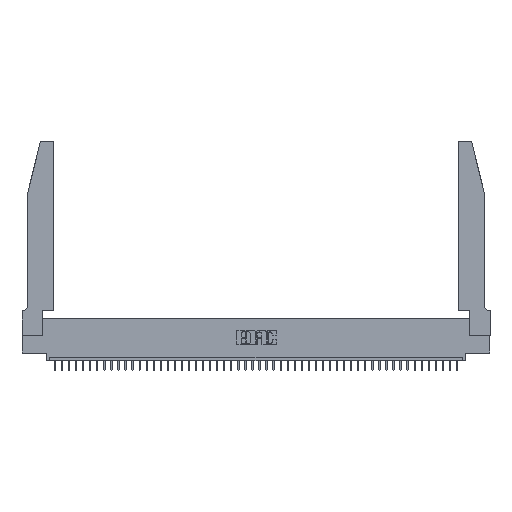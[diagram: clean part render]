
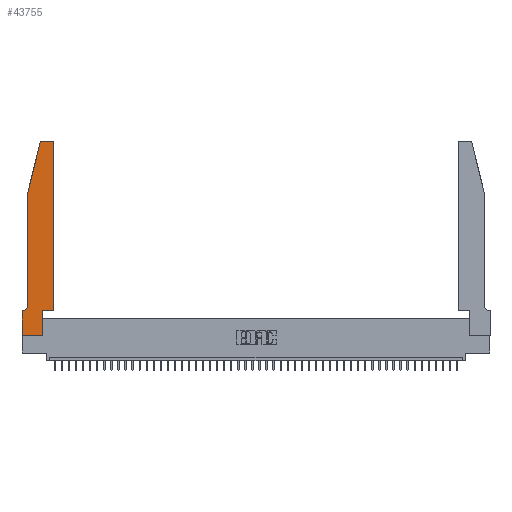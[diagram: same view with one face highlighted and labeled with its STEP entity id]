
A CAD part, top view. The second image highlights one B-rep face of the part: STEP entity #43755.
In plain terms, the highlighted planar face has unit normal (0, 0, 1).
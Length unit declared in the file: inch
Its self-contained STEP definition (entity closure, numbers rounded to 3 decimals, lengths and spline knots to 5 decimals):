
#264 = CARTESIAN_POINT ( 'NONE',  ( 0.4505, 0.35, 0.37 ) ) ;
#1302 = EDGE_CURVE ( 'NONE', #27855, #21250, #41207, .T. ) ;
#1537 = CARTESIAN_POINT ( 'NONE',  ( 0.2865, 0.35, 0.37 ) ) ;
#1675 = ORIENTED_EDGE ( 'NONE', *, *, #24866, .T. ) ;
#2288 = LINE ( 'NONE', #20576, #5714 ) ;
#2392 = ORIENTED_EDGE ( 'NONE', *, *, #37193, .T. ) ;
#2467 = DIRECTION ( 'NONE',  ( 1., 0., 0. ) ) ;
#2756 = DIRECTION ( 'NONE',  ( 0., 1., 0. ) ) ;
#2784 = CARTESIAN_POINT ( 'NONE',  ( 0., 0.35, 0.37 ) ) ;
#2833 = DIRECTION ( 'NONE',  ( 0., 1., 0. ) ) ;
#2867 = VERTEX_POINT ( 'NONE', #39076 ) ;
#2990 = LINE ( 'NONE', #38467, #31828 ) ;
#3200 = EDGE_CURVE ( 'NONE', #21250, #3592, #3771, .T. ) ;
#3344 = LINE ( 'NONE', #264, #46475 ) ;
#3357 = ORIENTED_EDGE ( 'NONE', *, *, #3200, .T. ) ;
#3592 = VERTEX_POINT ( 'NONE', #2784 ) ;
#3771 = LINE ( 'NONE', #38771, #34557 ) ;
#5037 = CARTESIAN_POINT ( 'NONE',  ( 0.0755, 2., 0.37 ) ) ;
#5418 = EDGE_CURVE ( 'NONE', #41456, #9614, #2288, .T. ) ;
#5714 = VECTOR ( 'NONE', #16613, 39.37008 ) ;
#5960 = LINE ( 'NONE', #45240, #11482 ) ;
#6958 = CARTESIAN_POINT ( 'NONE',  ( 0.284, 2.75, 0.37 ) ) ;
#9614 = VERTEX_POINT ( 'NONE', #36495 ) ;
#10933 = AXIS2_PLACEMENT_3D ( 'NONE', #23113, #23816, #38168 ) ;
#11343 = CIRCLE ( 'NONE', #37610, 0.03 ) ;
#11482 = VECTOR ( 'NONE', #2467, 39.37008 ) ;
#12267 = EDGE_LOOP ( 'NONE', ( #12749, #43530, #13342, #14851, #34036, #3357, #14149, #40280, #2392, #42584, #1675, #34532 ) ) ;
#12749 = ORIENTED_EDGE ( 'NONE', *, *, #28245, .T. ) ;
#12794 = EDGE_CURVE ( 'NONE', #17202, #34576, #3344, .T. ) ;
#12832 = AXIS2_PLACEMENT_3D ( 'NONE', #39432, #14291, #42969 ) ;
#13342 = ORIENTED_EDGE ( 'NONE', *, *, #5418, .T. ) ;
#13403 = VECTOR ( 'NONE', #40559, 39.37008 ) ;
#14149 = ORIENTED_EDGE ( 'NONE', *, *, #24190, .T. ) ;
#14291 = DIRECTION ( 'NONE',  ( 0., 0., 1. ) ) ;
#14851 = ORIENTED_EDGE ( 'NONE', *, *, #39822, .T. ) ;
#15056 = LINE ( 'NONE', #36428, #31975 ) ;
#16613 = DIRECTION ( 'NONE',  ( -0.239, -0.971, 0. ) ) ;
#17202 = VERTEX_POINT ( 'NONE', #1537 ) ;
#17816 = FACE_OUTER_BOUND ( 'NONE', #12267, .T. ) ;
#18684 = EDGE_CURVE ( 'NONE', #46118, #2867, #5960, .T. ) ;
#18891 = CARTESIAN_POINT ( 'NONE',  ( 0.0755, 0.42, 0.37 ) ) ;
#20576 = CARTESIAN_POINT ( 'NONE',  ( 0.0755, 2., 0.37 ) ) ;
#20604 = CARTESIAN_POINT ( 'NONE',  ( 0.4505, 0.35, 0.37 ) ) ;
#21250 = VERTEX_POINT ( 'NONE', #24347 ) ;
#21313 = VERTEX_POINT ( 'NONE', #6958 ) ;
#21409 = CARTESIAN_POINT ( 'NONE',  ( 0.2605, 2.75, 0.37 ) ) ;
#22088 = LINE ( 'NONE', #21409, #25911 ) ;
#22305 = DIRECTION ( 'NONE',  ( 0., -1., 0. ) ) ;
#23113 = CARTESIAN_POINT ( 'NONE',  ( 0.4205, 2.72, 0.37 ) ) ;
#23816 = DIRECTION ( 'NONE',  ( 0., 0., 1. ) ) ;
#24071 = EDGE_CURVE ( 'NONE', #45318, #38847, #34950, .T. ) ;
#24190 = EDGE_CURVE ( 'NONE', #3592, #46118, #15056, .T. ) ;
#24347 = CARTESIAN_POINT ( 'NONE',  ( 0.0055, 0.35, 0.37 ) ) ;
#24866 = EDGE_CURVE ( 'NONE', #34576, #45318, #2990, .T. ) ;
#25402 = DIRECTION ( 'NONE',  ( 1., 0., 0. ) ) ;
#25911 = VECTOR ( 'NONE', #35755, 39.37008 ) ;
#26119 = CARTESIAN_POINT ( 'NONE',  ( 0.4505, 2.72, 0.37 ) ) ;
#27855 = VERTEX_POINT ( 'NONE', #18891 ) ;
#28013 = CARTESIAN_POINT ( 'NONE',  ( 0.25487, 2.72718, 0.37 ) ) ;
#28245 = EDGE_CURVE ( 'NONE', #38847, #21313, #22088, .T. ) ;
#28891 = DIRECTION ( 'NONE',  ( -1., 0., 0. ) ) ;
#29204 = CARTESIAN_POINT ( 'NONE',  ( 0.4205, 2.75, 0.37 ) ) ;
#29949 = DIRECTION ( 'NONE',  ( -1., 0., 0. ) ) ;
#30561 = DIRECTION ( 'NONE',  ( 0., 0., 1. ) ) ;
#31332 = CARTESIAN_POINT ( 'NONE',  ( 0., 0., 0.37 ) ) ;
#31828 = VECTOR ( 'NONE', #2756, 39.37008 ) ;
#31975 = VECTOR ( 'NONE', #22305, 39.37008 ) ;
#34036 = ORIENTED_EDGE ( 'NONE', *, *, #1302, .T. ) ;
#34532 = ORIENTED_EDGE ( 'NONE', *, *, #24071, .T. ) ;
#34557 = VECTOR ( 'NONE', #28891, 39.37008 ) ;
#34576 = VERTEX_POINT ( 'NONE', #20604 ) ;
#34950 = CIRCLE ( 'NONE', #10933, 0.03 ) ;
#35016 = LINE ( 'NONE', #46083, #40634 ) ;
#35755 = DIRECTION ( 'NONE',  ( -1., 0., 0. ) ) ;
#36428 = CARTESIAN_POINT ( 'NONE',  ( 0., 0., 0.37 ) ) ;
#36495 = CARTESIAN_POINT ( 'NONE',  ( 0.0755, 2., 0.37 ) ) ;
#36989 = CARTESIAN_POINT ( 'NONE',  ( 0.0055, 0.42, 0.37 ) ) ;
#37030 = EDGE_CURVE ( 'NONE', #21313, #41456, #11343, .T. ) ;
#37193 = EDGE_CURVE ( 'NONE', #2867, #17202, #35016, .T. ) ;
#37380 = CARTESIAN_POINT ( 'NONE',  ( 0.284, 2.72, 0.37 ) ) ;
#37610 = AXIS2_PLACEMENT_3D ( 'NONE', #37380, #30561, #44678 ) ;
#38168 = DIRECTION ( 'NONE',  ( 1., 0., 0. ) ) ;
#38467 = CARTESIAN_POINT ( 'NONE',  ( 0.4505, 0.35, 0.37 ) ) ;
#38771 = CARTESIAN_POINT ( 'NONE',  ( 0.0755, 0.35, 0.37 ) ) ;
#38847 = VERTEX_POINT ( 'NONE', #29204 ) ;
#39076 = CARTESIAN_POINT ( 'NONE',  ( 0.2865, 0., 0.37 ) ) ;
#39432 = CARTESIAN_POINT ( 'NONE',  ( 0., 0.35, 0.37 ) ) ;
#39658 = PLANE ( 'NONE',  #12832 ) ;
#39822 = EDGE_CURVE ( 'NONE', #9614, #27855, #44765, .T. ) ;
#40280 = ORIENTED_EDGE ( 'NONE', *, *, #18684, .T. ) ;
#40559 = DIRECTION ( 'NONE',  ( 0., -1., 0. ) ) ;
#40634 = VECTOR ( 'NONE', #2833, 39.37008 ) ;
#41207 = CIRCLE ( 'NONE', #44224, 0.07 ) ;
#41456 = VERTEX_POINT ( 'NONE', #28013 ) ;
#42584 = ORIENTED_EDGE ( 'NONE', *, *, #12794, .T. ) ;
#42969 = DIRECTION ( 'NONE',  ( 1., 0., 0. ) ) ;
#43530 = ORIENTED_EDGE ( 'NONE', *, *, #37030, .T. ) ;
#43755 = ADVANCED_FACE ( 'NONE', ( #17816 ), #39658, .T. ) ;
#44224 = AXIS2_PLACEMENT_3D ( 'NONE', #36989, #44533, #29949 ) ;
#44533 = DIRECTION ( 'NONE',  ( 0., 0., -1. ) ) ;
#44678 = DIRECTION ( 'NONE',  ( 1., 0., 0. ) ) ;
#44765 = LINE ( 'NONE', #5037, #13403 ) ;
#45240 = CARTESIAN_POINT ( 'NONE',  ( 0., 0., 0.37 ) ) ;
#45318 = VERTEX_POINT ( 'NONE', #26119 ) ;
#46083 = CARTESIAN_POINT ( 'NONE',  ( 0.2865, 0.35, 0.37 ) ) ;
#46118 = VERTEX_POINT ( 'NONE', #31332 ) ;
#46475 = VECTOR ( 'NONE', #25402, 39.37008 ) ;
